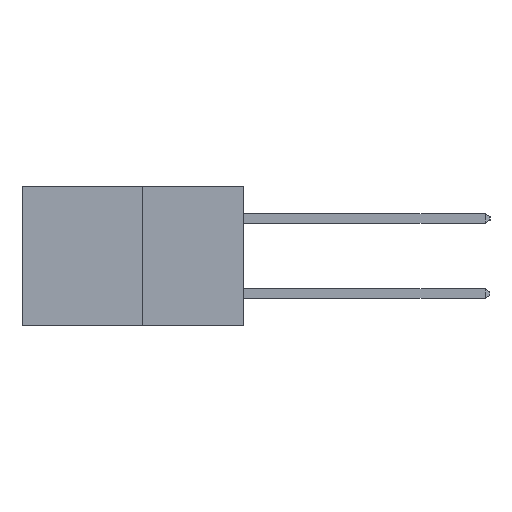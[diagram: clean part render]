
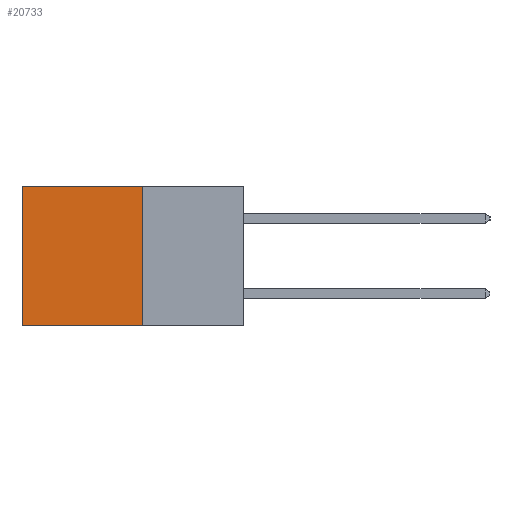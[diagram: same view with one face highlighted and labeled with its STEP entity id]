
A CAD part, left-side view. The second image highlights one B-rep face of the part: STEP entity #20733.
In plain terms, the highlighted planar face has unit normal (-1, 0, 0).
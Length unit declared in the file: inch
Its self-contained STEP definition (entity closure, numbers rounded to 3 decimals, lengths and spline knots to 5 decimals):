
#819 = LINE ( 'NONE', #10430, #5697 ) ;
#1284 = PLANE ( 'NONE',  #18068 ) ;
#1292 = EDGE_LOOP ( 'NONE', ( #2724, #19187, #21851, #13965 ) ) ;
#1520 = DIRECTION ( 'NONE',  ( 0., 0., -1. ) ) ;
#1823 = DIRECTION ( 'NONE',  ( 0., 0., -1. ) ) ;
#2146 = LINE ( 'NONE', #11931, #21018 ) ;
#2724 = ORIENTED_EDGE ( 'NONE', *, *, #14256, .T. ) ;
#3020 = DIRECTION ( 'NONE',  ( 0., 1., 0. ) ) ;
#3125 = CARTESIAN_POINT ( 'NONE',  ( 0.277, 0.27, -0.37 ) ) ;
#3398 = VECTOR ( 'NONE', #4787, 39.37008 ) ;
#4787 = DIRECTION ( 'NONE',  ( 0., 1., 0. ) ) ;
#4970 = DIRECTION ( 'NONE',  ( 1., 0., 0. ) ) ;
#5135 = VERTEX_POINT ( 'NONE', #20443 ) ;
#5697 = VECTOR ( 'NONE', #1520, 39.37008 ) ;
#6414 = VERTEX_POINT ( 'NONE', #8040 ) ;
#7777 = EDGE_CURVE ( 'NONE', #6414, #10115, #2146, .T. ) ;
#8040 = CARTESIAN_POINT ( 'NONE',  ( 0.277, 0.27, 0. ) ) ;
#9009 = CARTESIAN_POINT ( 'NONE',  ( 0.277, 0.59, -0.37 ) ) ;
#10115 = VERTEX_POINT ( 'NONE', #13580 ) ;
#10430 = CARTESIAN_POINT ( 'NONE',  ( 0.277, 0.27, -0.37 ) ) ;
#11931 = CARTESIAN_POINT ( 'NONE',  ( 0.277, 0.27, 0. ) ) ;
#12899 = VERTEX_POINT ( 'NONE', #19375 ) ;
#13440 = LINE ( 'NONE', #22269, #3398 ) ;
#13580 = CARTESIAN_POINT ( 'NONE',  ( 0.277, 0.59, 0. ) ) ;
#13965 = ORIENTED_EDGE ( 'NONE', *, *, #7777, .T. ) ;
#14256 = EDGE_CURVE ( 'NONE', #10115, #5135, #21856, .T. ) ;
#16239 = FACE_OUTER_BOUND ( 'NONE', #1292, .T. ) ;
#17242 = VECTOR ( 'NONE', #1823, 39.37008 ) ;
#17382 = DIRECTION ( 'NONE',  ( 0., 0., -1. ) ) ;
#18068 = AXIS2_PLACEMENT_3D ( 'NONE', #3125, #4970, #17382 ) ;
#19187 = ORIENTED_EDGE ( 'NONE', *, *, #21315, .F. ) ;
#19375 = CARTESIAN_POINT ( 'NONE',  ( 0.277, 0.27, -0.37 ) ) ;
#20443 = CARTESIAN_POINT ( 'NONE',  ( 0.277, 0.59, -0.37 ) ) ;
#20733 = ADVANCED_FACE ( 'NONE', ( #16239 ), #1284, .F. ) ;
#20813 = EDGE_CURVE ( 'NONE', #6414, #12899, #819, .T. ) ;
#21018 = VECTOR ( 'NONE', #3020, 39.37008 ) ;
#21315 = EDGE_CURVE ( 'NONE', #12899, #5135, #13440, .T. ) ;
#21851 = ORIENTED_EDGE ( 'NONE', *, *, #20813, .F. ) ;
#21856 = LINE ( 'NONE', #9009, #17242 ) ;
#22269 = CARTESIAN_POINT ( 'NONE',  ( 0.277, 0.27, -0.37 ) ) ;
